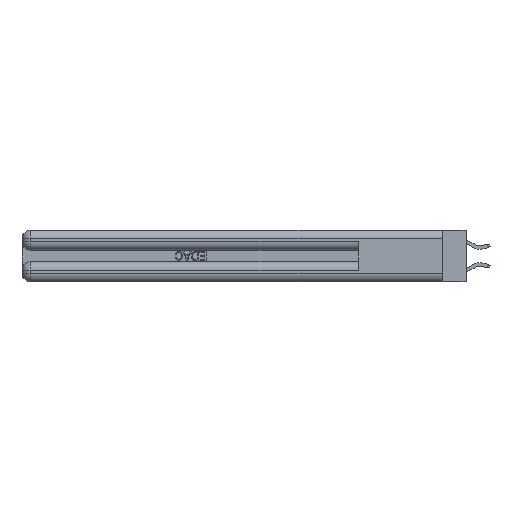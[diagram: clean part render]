
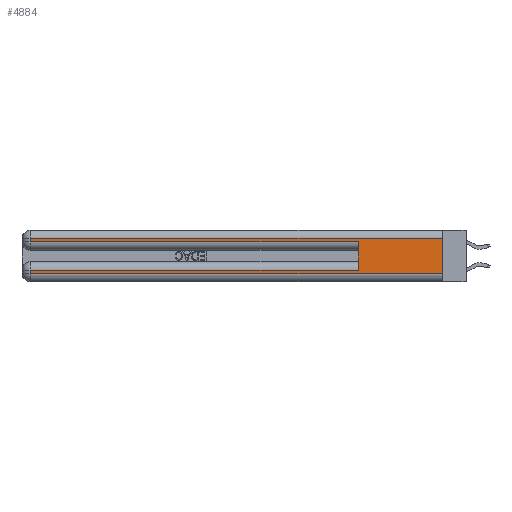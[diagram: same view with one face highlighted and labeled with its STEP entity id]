
A CAD part, left-side view. The second image highlights one B-rep face of the part: STEP entity #4884.
In plain terms, the highlighted planar face has unit normal (-1, 0, 0).
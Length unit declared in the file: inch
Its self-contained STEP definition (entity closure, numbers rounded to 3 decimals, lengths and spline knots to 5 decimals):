
#104 = EDGE_CURVE ( 'NONE', #30187, #31951, #20009, .T. ) ;
#295 = DIRECTION ( 'NONE',  ( 0., 1., 0. ) ) ;
#852 = VECTOR ( 'NONE', #17271, 39.37008 ) ;
#993 = DIRECTION ( 'NONE',  ( 0., -1., 0. ) ) ;
#1148 = DIRECTION ( 'NONE',  ( 0., 0., -1. ) ) ;
#1554 = CARTESIAN_POINT ( 'NONE',  ( 0., 2.94, 0.285 ) ) ;
#4884 = ADVANCED_FACE ( 'NONE', ( #21163 ), #18251, .F. ) ;
#5824 = AXIS2_PLACEMENT_3D ( 'NONE', #7327, #26111, #1148 ) ;
#6950 = DIRECTION ( 'NONE',  ( 0., 0., -1. ) ) ;
#7327 = CARTESIAN_POINT ( 'NONE',  ( 0., 0., 0.37 ) ) ;
#8671 = LINE ( 'NONE', #28316, #35003 ) ;
#9034 = ORIENTED_EDGE ( 'NONE', *, *, #17024, .T. ) ;
#9515 = LINE ( 'NONE', #29338, #19667 ) ;
#10515 = CARTESIAN_POINT ( 'NONE',  ( 0., 0., 0.31 ) ) ;
#11444 = CARTESIAN_POINT ( 'NONE',  ( 0., 0., 0.285 ) ) ;
#13453 = ORIENTED_EDGE ( 'NONE', *, *, #13951, .F. ) ;
#13568 = VECTOR ( 'NONE', #34036, 39.37008 ) ;
#13951 = EDGE_CURVE ( 'NONE', #29336, #22955, #15547, .T. ) ;
#15045 = VECTOR ( 'NONE', #22122, 39.37008 ) ;
#15547 = LINE ( 'NONE', #18267, #16870 ) ;
#16870 = VECTOR ( 'NONE', #29382, 39.37008 ) ;
#17024 = EDGE_CURVE ( 'NONE', #23671, #30083, #22872, .T. ) ;
#17037 = ORIENTED_EDGE ( 'NONE', *, *, #20968, .F. ) ;
#17271 = DIRECTION ( 'NONE',  ( 0., -1., 0. ) ) ;
#17578 = CARTESIAN_POINT ( 'NONE',  ( 0., 0., 0.06 ) ) ;
#17729 = EDGE_CURVE ( 'NONE', #31951, #22955, #25293, .T. ) ;
#18251 = PLANE ( 'NONE',  #5824 ) ;
#18267 = CARTESIAN_POINT ( 'NONE',  ( 0., 0.6, 0.145 ) ) ;
#19442 = CARTESIAN_POINT ( 'NONE',  ( 0., 2.94, 0.06 ) ) ;
#19667 = VECTOR ( 'NONE', #6950, 39.37008 ) ;
#19707 = CARTESIAN_POINT ( 'NONE',  ( 0., 0.6, 0.085 ) ) ;
#19769 = DIRECTION ( 'NONE',  ( 0., 0., -1. ) ) ;
#20009 = LINE ( 'NONE', #31138, #13568 ) ;
#20398 = EDGE_CURVE ( 'NONE', #35883, #30187, #25223, .T. ) ;
#20443 = CARTESIAN_POINT ( 'NONE',  ( 0., 0.6, 0.285 ) ) ;
#20830 = LINE ( 'NONE', #29211, #34971 ) ;
#20968 = EDGE_CURVE ( 'NONE', #35883, #30083, #9515, .T. ) ;
#21163 = FACE_OUTER_BOUND ( 'NONE', #34696, .T. ) ;
#21401 = CARTESIAN_POINT ( 'NONE',  ( 0., 0., 0.06 ) ) ;
#22122 = DIRECTION ( 'NONE',  ( 0., 1., 0. ) ) ;
#22453 = EDGE_CURVE ( 'NONE', #29336, #33211, #20830, .T. ) ;
#22872 = LINE ( 'NONE', #17578, #26869 ) ;
#22955 = VERTEX_POINT ( 'NONE', #20443 ) ;
#23286 = ORIENTED_EDGE ( 'NONE', *, *, #17729, .T. ) ;
#23671 = VERTEX_POINT ( 'NONE', #19442 ) ;
#23764 = ORIENTED_EDGE ( 'NONE', *, *, #104, .T. ) ;
#23931 = ORIENTED_EDGE ( 'NONE', *, *, #24274, .T. ) ;
#24274 = EDGE_CURVE ( 'NONE', #33211, #23671, #8671, .T. ) ;
#24519 = ORIENTED_EDGE ( 'NONE', *, *, #22453, .T. ) ;
#24685 = CARTESIAN_POINT ( 'NONE',  ( 0., 0., 0.31 ) ) ;
#25223 = LINE ( 'NONE', #24685, #15045 ) ;
#25293 = LINE ( 'NONE', #11444, #852 ) ;
#26111 = DIRECTION ( 'NONE',  ( 1., 0., 0. ) ) ;
#26834 = ORIENTED_EDGE ( 'NONE', *, *, #20398, .T. ) ;
#26869 = VECTOR ( 'NONE', #993, 39.37008 ) ;
#28221 = CARTESIAN_POINT ( 'NONE',  ( 0., 2.94, 0.085 ) ) ;
#28316 = CARTESIAN_POINT ( 'NONE',  ( 0., 2.94, 0.37 ) ) ;
#29211 = CARTESIAN_POINT ( 'NONE',  ( 0., 0., 0.085 ) ) ;
#29336 = VERTEX_POINT ( 'NONE', #19707 ) ;
#29338 = CARTESIAN_POINT ( 'NONE',  ( 0., 0., 0.37 ) ) ;
#29382 = DIRECTION ( 'NONE',  ( 0., 0., 1. ) ) ;
#30083 = VERTEX_POINT ( 'NONE', #21401 ) ;
#30187 = VERTEX_POINT ( 'NONE', #33784 ) ;
#31138 = CARTESIAN_POINT ( 'NONE',  ( 0., 2.94, 0.37 ) ) ;
#31951 = VERTEX_POINT ( 'NONE', #1554 ) ;
#33211 = VERTEX_POINT ( 'NONE', #28221 ) ;
#33784 = CARTESIAN_POINT ( 'NONE',  ( 0., 2.94, 0.31 ) ) ;
#34036 = DIRECTION ( 'NONE',  ( 0., 0., -1. ) ) ;
#34696 = EDGE_LOOP ( 'NONE', ( #17037, #26834, #23764, #23286, #13453, #24519, #23931, #9034 ) ) ;
#34971 = VECTOR ( 'NONE', #295, 39.37008 ) ;
#35003 = VECTOR ( 'NONE', #19769, 39.37008 ) ;
#35883 = VERTEX_POINT ( 'NONE', #10515 ) ;
